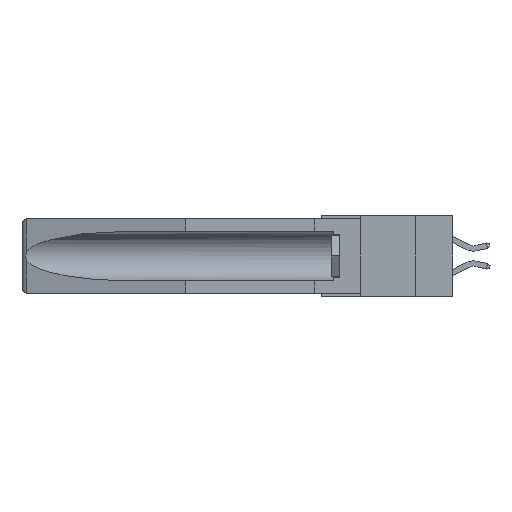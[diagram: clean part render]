
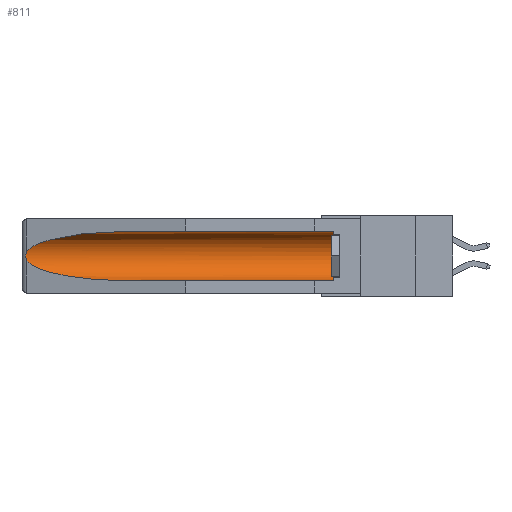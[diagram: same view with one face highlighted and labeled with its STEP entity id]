
A CAD part, left-side view. The second image highlights one B-rep face of the part: STEP entity #811.
In plain terms, the highlighted cylindrical face has radius 2.857 mm (diameter 5.715 mm), a partial arc.
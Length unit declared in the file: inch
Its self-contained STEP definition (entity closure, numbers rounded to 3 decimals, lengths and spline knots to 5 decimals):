
#811 = ADVANCED_FACE ( 'NONE', ( #20342 ), #13638, .F. ) ;
#864 = CARTESIAN_POINT ( 'NONE',  ( 0.26597, 1.5296, -0.19026 ) ) ;
#983 = CARTESIAN_POINT ( 'NONE',  ( 0.2675, 1.53308, -0.16763 ) ) ;
#1756 = LINE ( 'NONE', #6453, #6829 ) ;
#2202 = VECTOR ( 'NONE', #29094, 39.37008 ) ;
#3650 = CARTESIAN_POINT ( 'NONE',  ( 0.25451, 1.48313, -0.24835 ) ) ;
#3846 = ORIENTED_EDGE ( 'NONE', *, *, #26264, .T. ) ;
#4779 = CARTESIAN_POINT ( 'NONE',  ( 0.155, -0.30754, -0.284 ) ) ;
#5360 = CARTESIAN_POINT ( 'NONE',  ( 0.155, 0.126, -0.1715 ) ) ;
#6384 = CARTESIAN_POINT ( 'NONE',  ( 0.2673, 1.5327, -0.16383 ) ) ;
#6453 = CARTESIAN_POINT ( 'NONE',  ( 0.155, -0.30754, -0.059 ) ) ;
#6788 = VERTEX_POINT ( 'NONE', #13784 ) ;
#6829 = VECTOR ( 'NONE', #22616, 39.37008 ) ;
#7025 = ORIENTED_EDGE ( 'NONE', *, *, #12767, .T. ) ;
#8656 = EDGE_LOOP ( 'NONE', ( #7025, #3846, #16964, #28912, #24903, #13575 ) ) ;
#8718 = CARTESIAN_POINT ( 'NONE',  ( 0.26537, 1.52718, -0.14972 ) ) ;
#8837 = CARTESIAN_POINT ( 'NONE',  ( 0.26597, 1.52961, -0.15275 ) ) ;
#9460 = DIRECTION ( 'NONE',  ( 0., 1., 0. ) ) ;
#9804 = EDGE_CURVE ( 'NONE', #30091, #20597, #26017, .T. ) ;
#10605 = DIRECTION ( 'NONE',  ( 0., -1., 0. ) ) ;
#11136 = CARTESIAN_POINT ( 'NONE',  ( 0.155, 1.07973, -0.059 ) ) ;
#11506 = CARTESIAN_POINT ( 'NONE',  ( 0.26654, 1.53092, -0.15636 ) ) ;
#12748 = CARTESIAN_POINT ( 'NONE',  ( 0.155, 1.07973, -0.059 ) ) ;
#12767 = EDGE_CURVE ( 'NONE', #20856, #6788, #20841, .T. ) ;
#13575 = ORIENTED_EDGE ( 'NONE', *, *, #27645, .T. ) ;
#13638 = CYLINDRICAL_SURFACE ( 'NONE', #24169, 0.1125 ) ;
#13784 = CARTESIAN_POINT ( 'NONE',  ( 0.26537, 1.52718, -0.14972 ) ) ;
#14057 = AXIS2_PLACEMENT_3D ( 'NONE', #5360, #10605, #27170 ) ;
#14092 = VERTEX_POINT ( 'NONE', #26756 ) ;
#14188 = CARTESIAN_POINT ( 'NONE',  ( 0.26537, 1.52718, -0.14972 ) ) ;
#14923 = CARTESIAN_POINT ( 'NONE',  ( 0.26537, 1.52718, -0.19328 ) ) ;
#16294 = VERTEX_POINT ( 'NONE', #25226 ) ;
#16565 = B_SPLINE_CURVE_WITH_KNOTS ( 'NONE', 3,
 ( #8718, #8837, #11506, #6384, #983, #22322, #24799, #19756, #864, #27730 ),
 .UNSPECIFIED., .F., .F.,
 ( 4, 2, 2, 2, 4 ),
 ( 0., 0.00029, 0.00058, 0.00087, 0.00117 ),
 .UNSPECIFIED. ) ;
#16964 = ORIENTED_EDGE ( 'NONE', *, *, #9804, .T. ) ;
#19741 = CARTESIAN_POINT ( 'NONE',  ( 0.26537, 1.52718, -0.19328 ) ) ;
#19756 = CARTESIAN_POINT ( 'NONE',  ( 0.26655, 1.53094, -0.18657 ) ) ;
#20016 = CARTESIAN_POINT ( 'NONE',  ( 0.155, -0.30754, -0.1715 ) ) ;
#20342 = FACE_OUTER_BOUND ( 'NONE', #8656, .T. ) ;
#20597 = VERTEX_POINT ( 'NONE', #25804 ) ;
#20841 =( BOUNDED_CURVE ( )  B_SPLINE_CURVE ( 3, ( #11136, #24873, #29935, #14188 ),
 .UNSPECIFIED., .F., .F. ) 
 B_SPLINE_CURVE_WITH_KNOTS ( ( 4, 4 ),
 ( 4.71239, 6.08839 ),
 .UNSPECIFIED. ) 
 CURVE ( )  GEOMETRIC_REPRESENTATION_ITEM ( )  RATIONAL_B_SPLINE_CURVE ( ( 1., 0.848, 0.848, 1. ) ) 
 REPRESENTATION_ITEM ( '' )  );
#20856 = VERTEX_POINT ( 'NONE', #12748 ) ;
#21934 = LINE ( 'NONE', #4779, #2202 ) ;
#22322 = CARTESIAN_POINT ( 'NONE',  ( 0.2675, 1.53308, -0.17534 ) ) ;
#22616 = DIRECTION ( 'NONE',  ( 0., 1., 0. ) ) ;
#24169 = AXIS2_PLACEMENT_3D ( 'NONE', #20016, #9460, #33985 ) ;
#24799 = CARTESIAN_POINT ( 'NONE',  ( 0.2673, 1.53269, -0.17917 ) ) ;
#24873 = CARTESIAN_POINT ( 'NONE',  ( 0.21114, 1.30732, -0.059 ) ) ;
#24903 = ORIENTED_EDGE ( 'NONE', *, *, #31596, .T. ) ;
#25226 = CARTESIAN_POINT ( 'NONE',  ( 0.155, 0.126, -0.284 ) ) ;
#25804 = CARTESIAN_POINT ( 'NONE',  ( 0.155, 1.07973, -0.284 ) ) ;
#26017 =( BOUNDED_CURVE ( )  B_SPLINE_CURVE ( 3, ( #19741, #3650, #30539, #33246 ),
 .UNSPECIFIED., .F., .F. ) 
 B_SPLINE_CURVE_WITH_KNOTS ( ( 4, 4 ),
 ( 0.1948, 1.5708 ),
 .UNSPECIFIED. ) 
 CURVE ( )  GEOMETRIC_REPRESENTATION_ITEM ( )  RATIONAL_B_SPLINE_CURVE ( ( 1., 0.848, 0.848, 1. ) ) 
 REPRESENTATION_ITEM ( '' )  );
#26264 = EDGE_CURVE ( 'NONE', #6788, #30091, #16565, .T. ) ;
#26756 = CARTESIAN_POINT ( 'NONE',  ( 0.155, 0.126, -0.059 ) ) ;
#27170 = DIRECTION ( 'NONE',  ( 0., 0., 1. ) ) ;
#27645 = EDGE_CURVE ( 'NONE', #14092, #20856, #1756, .T. ) ;
#27730 = CARTESIAN_POINT ( 'NONE',  ( 0.26537, 1.52718, -0.19328 ) ) ;
#28912 = ORIENTED_EDGE ( 'NONE', *, *, #30902, .F. ) ;
#29094 = DIRECTION ( 'NONE',  ( 0., 1., 0. ) ) ;
#29935 = CARTESIAN_POINT ( 'NONE',  ( 0.25451, 1.48313, -0.09465 ) ) ;
#30091 = VERTEX_POINT ( 'NONE', #14923 ) ;
#30539 = CARTESIAN_POINT ( 'NONE',  ( 0.21114, 1.30732, -0.284 ) ) ;
#30902 = EDGE_CURVE ( 'NONE', #16294, #20597, #21934, .T. ) ;
#31596 = EDGE_CURVE ( 'NONE', #16294, #14092, #33245, .T. ) ;
#33245 = CIRCLE ( 'NONE', #14057, 0.1125 ) ;
#33246 = CARTESIAN_POINT ( 'NONE',  ( 0.155, 1.07973, -0.284 ) ) ;
#33985 = DIRECTION ( 'NONE',  ( 0., 0., 1. ) ) ;
